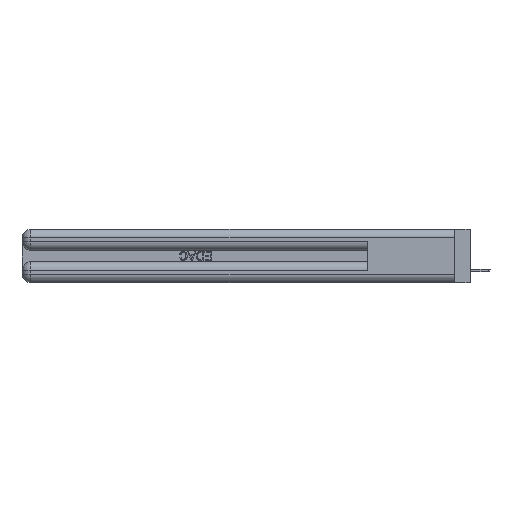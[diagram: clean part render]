
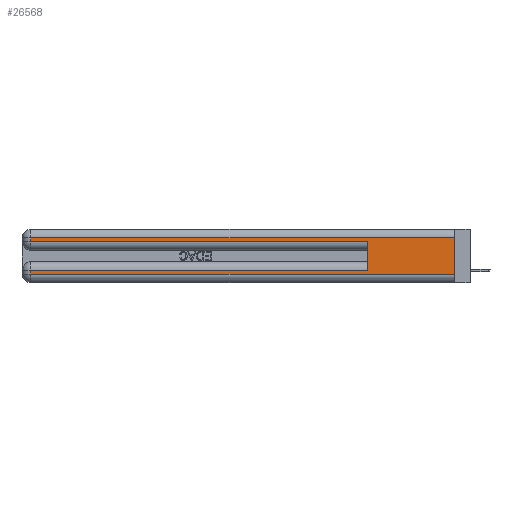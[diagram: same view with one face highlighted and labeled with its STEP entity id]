
A CAD part, left-side view. The second image highlights one B-rep face of the part: STEP entity #26568.
In plain terms, the highlighted planar face has unit normal (-1, 0, 0).
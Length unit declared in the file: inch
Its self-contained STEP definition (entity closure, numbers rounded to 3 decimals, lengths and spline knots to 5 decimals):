
#827 = CARTESIAN_POINT ( 'NONE',  ( 0., 0., 0.06 ) ) ;
#2557 = VECTOR ( 'NONE', #37872, 39.37008 ) ;
#3969 = VERTEX_POINT ( 'NONE', #9774 ) ;
#5605 = CARTESIAN_POINT ( 'NONE',  ( 0., 0., 0.37 ) ) ;
#5792 = DIRECTION ( 'NONE',  ( 0., 0., -1. ) ) ;
#6025 = DIRECTION ( 'NONE',  ( 0., 0., -1. ) ) ;
#6538 = ORIENTED_EDGE ( 'NONE', *, *, #18907, .T. ) ;
#6693 = EDGE_CURVE ( 'NONE', #3969, #7624, #37822, .T. ) ;
#7329 = EDGE_CURVE ( 'NONE', #27174, #3969, #25691, .T. ) ;
#7428 = CARTESIAN_POINT ( 'NONE',  ( 0., 0., 0.06 ) ) ;
#7624 = VERTEX_POINT ( 'NONE', #34003 ) ;
#7651 = EDGE_CURVE ( 'NONE', #41860, #21792, #11893, .T. ) ;
#9647 = CARTESIAN_POINT ( 'NONE',  ( 0., 0.6, 0.085 ) ) ;
#9774 = CARTESIAN_POINT ( 'NONE',  ( 0., 2.94, 0.285 ) ) ;
#11006 = LINE ( 'NONE', #23905, #11612 ) ;
#11359 = EDGE_CURVE ( 'NONE', #17779, #41860, #16257, .T. ) ;
#11612 = VECTOR ( 'NONE', #20848, 39.37008 ) ;
#11893 = LINE ( 'NONE', #25858, #36025 ) ;
#12487 = ORIENTED_EDGE ( 'NONE', *, *, #11359, .T. ) ;
#13482 = ORIENTED_EDGE ( 'NONE', *, *, #22809, .F. ) ;
#14017 = VECTOR ( 'NONE', #15393, 39.37008 ) ;
#14228 = AXIS2_PLACEMENT_3D ( 'NONE', #16035, #22594, #6025 ) ;
#14649 = EDGE_CURVE ( 'NONE', #17779, #7624, #20792, .T. ) ;
#15393 = DIRECTION ( 'NONE',  ( 0., 0., -1. ) ) ;
#15858 = EDGE_CURVE ( 'NONE', #42315, #27174, #11006, .T. ) ;
#16035 = CARTESIAN_POINT ( 'NONE',  ( 0., 0., 0.37 ) ) ;
#16257 = LINE ( 'NONE', #29618, #40711 ) ;
#17656 = LINE ( 'NONE', #7428, #27102 ) ;
#17779 = VERTEX_POINT ( 'NONE', #9647 ) ;
#18907 = EDGE_CURVE ( 'NONE', #21792, #20555, #17656, .T. ) ;
#20555 = VERTEX_POINT ( 'NONE', #827 ) ;
#20792 = LINE ( 'NONE', #21414, #2557 ) ;
#20848 = DIRECTION ( 'NONE',  ( 0., 1., 0. ) ) ;
#21414 = CARTESIAN_POINT ( 'NONE',  ( 0., 0.6, 0.145 ) ) ;
#21792 = VERTEX_POINT ( 'NONE', #40522 ) ;
#21803 = DIRECTION ( 'NONE',  ( 0., -1., 0. ) ) ;
#22150 = FACE_OUTER_BOUND ( 'NONE', #29561, .T. ) ;
#22236 = VECTOR ( 'NONE', #35783, 39.37008 ) ;
#22594 = DIRECTION ( 'NONE',  ( 1., 0., 0. ) ) ;
#22809 = EDGE_CURVE ( 'NONE', #42315, #20555, #28082, .T. ) ;
#23905 = CARTESIAN_POINT ( 'NONE',  ( 0., 0., 0.31 ) ) ;
#25691 = LINE ( 'NONE', #35557, #22236 ) ;
#25858 = CARTESIAN_POINT ( 'NONE',  ( 0., 2.94, 0.37 ) ) ;
#26515 = CARTESIAN_POINT ( 'NONE',  ( 0., 0., 0.31 ) ) ;
#26568 = ADVANCED_FACE ( 'NONE', ( #22150 ), #28959, .F. ) ;
#27102 = VECTOR ( 'NONE', #27498, 39.37008 ) ;
#27174 = VERTEX_POINT ( 'NONE', #34931 ) ;
#27498 = DIRECTION ( 'NONE',  ( 0., -1., 0. ) ) ;
#28082 = LINE ( 'NONE', #5605, #14017 ) ;
#28959 = PLANE ( 'NONE',  #14228 ) ;
#29432 = CARTESIAN_POINT ( 'NONE',  ( 0., 2.94, 0.085 ) ) ;
#29561 = EDGE_LOOP ( 'NONE', ( #13482, #38998, #38996, #37756, #31149, #12487, #36350, #6538 ) ) ;
#29618 = CARTESIAN_POINT ( 'NONE',  ( 0., 0., 0.085 ) ) ;
#31149 = ORIENTED_EDGE ( 'NONE', *, *, #14649, .F. ) ;
#32701 = VECTOR ( 'NONE', #21803, 39.37008 ) ;
#33120 = DIRECTION ( 'NONE',  ( 0., 1., 0. ) ) ;
#34003 = CARTESIAN_POINT ( 'NONE',  ( 0., 0.6, 0.285 ) ) ;
#34931 = CARTESIAN_POINT ( 'NONE',  ( 0., 2.94, 0.31 ) ) ;
#35178 = CARTESIAN_POINT ( 'NONE',  ( 0., 0., 0.285 ) ) ;
#35557 = CARTESIAN_POINT ( 'NONE',  ( 0., 2.94, 0.37 ) ) ;
#35783 = DIRECTION ( 'NONE',  ( 0., 0., -1. ) ) ;
#36025 = VECTOR ( 'NONE', #5792, 39.37008 ) ;
#36350 = ORIENTED_EDGE ( 'NONE', *, *, #7651, .T. ) ;
#37756 = ORIENTED_EDGE ( 'NONE', *, *, #6693, .T. ) ;
#37822 = LINE ( 'NONE', #35178, #32701 ) ;
#37872 = DIRECTION ( 'NONE',  ( 0., 0., 1. ) ) ;
#38996 = ORIENTED_EDGE ( 'NONE', *, *, #7329, .T. ) ;
#38998 = ORIENTED_EDGE ( 'NONE', *, *, #15858, .T. ) ;
#40522 = CARTESIAN_POINT ( 'NONE',  ( 0., 2.94, 0.06 ) ) ;
#40711 = VECTOR ( 'NONE', #33120, 39.37008 ) ;
#41860 = VERTEX_POINT ( 'NONE', #29432 ) ;
#42315 = VERTEX_POINT ( 'NONE', #26515 ) ;
